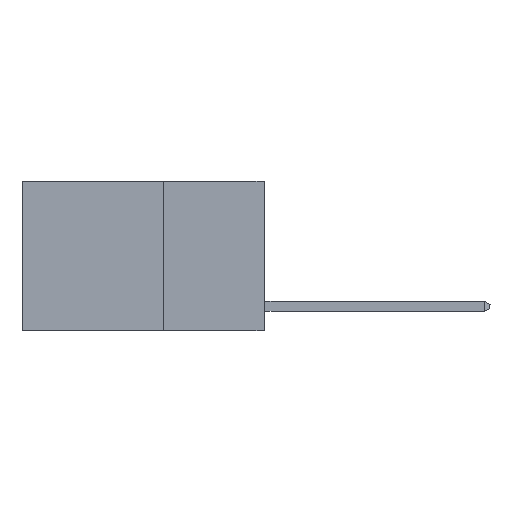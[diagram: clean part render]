
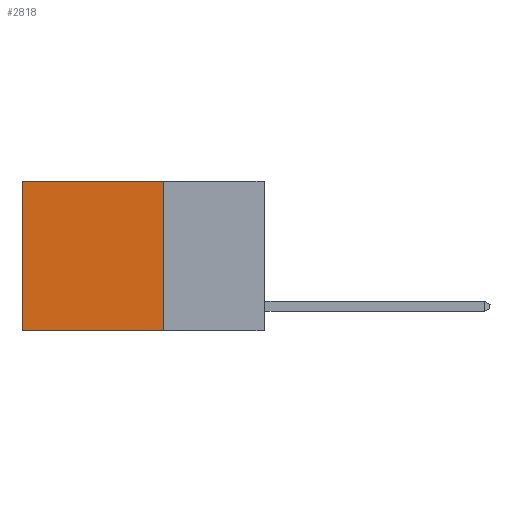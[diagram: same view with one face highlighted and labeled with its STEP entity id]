
A CAD part, left-side view. The second image highlights one B-rep face of the part: STEP entity #2818.
In plain terms, the highlighted planar face has unit normal (-1, 0, 0).
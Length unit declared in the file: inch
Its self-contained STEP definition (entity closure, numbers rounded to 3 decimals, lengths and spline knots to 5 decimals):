
#134 = VECTOR ( 'NONE', #1135, 39.37008 ) ;
#278 = VERTEX_POINT ( 'NONE', #2624 ) ;
#439 = EDGE_CURVE ( 'NONE', #278, #7515, #12090, .T. ) ;
#1135 = DIRECTION ( 'NONE',  ( 0., 1., 0. ) ) ;
#1169 = DIRECTION ( 'NONE',  ( 0., 0., -1. ) ) ;
#2047 = CARTESIAN_POINT ( 'NONE',  ( 0.2625, 0.6, 0. ) ) ;
#2213 = CARTESIAN_POINT ( 'NONE',  ( 0.2625, 0.25, -0.37 ) ) ;
#2285 = ORIENTED_EDGE ( 'NONE', *, *, #439, .F. ) ;
#2624 = CARTESIAN_POINT ( 'NONE',  ( 0.2625, 0.25, -0.37 ) ) ;
#2818 = ADVANCED_FACE ( 'NONE', ( #10756 ), #8108, .F. ) ;
#3013 = VECTOR ( 'NONE', #17238, 39.37008 ) ;
#3111 = VERTEX_POINT ( 'NONE', #2047 ) ;
#3143 = ORIENTED_EDGE ( 'NONE', *, *, #16638, .T. ) ;
#3815 = CARTESIAN_POINT ( 'NONE',  ( 0.2625, 0.25, 0. ) ) ;
#5199 = CARTESIAN_POINT ( 'NONE',  ( 0.2625, 0.25, 0. ) ) ;
#5570 = EDGE_LOOP ( 'NONE', ( #3143, #2285, #6544, #8696 ) ) ;
#6138 = AXIS2_PLACEMENT_3D ( 'NONE', #5199, #16607, #16341 ) ;
#6544 = ORIENTED_EDGE ( 'NONE', *, *, #11732, .F. ) ;
#7515 = VERTEX_POINT ( 'NONE', #16007 ) ;
#8108 = PLANE ( 'NONE',  #6138 ) ;
#8696 = ORIENTED_EDGE ( 'NONE', *, *, #10519, .T. ) ;
#9375 = DIRECTION ( 'NONE',  ( 0., 1., 0. ) ) ;
#10280 = LINE ( 'NONE', #11666, #3013 ) ;
#10519 = EDGE_CURVE ( 'NONE', #14556, #3111, #14672, .T. ) ;
#10756 = FACE_OUTER_BOUND ( 'NONE', #5570, .T. ) ;
#11666 = CARTESIAN_POINT ( 'NONE',  ( 0.2625, 0.6, 0. ) ) ;
#11732 = EDGE_CURVE ( 'NONE', #14556, #278, #17517, .T. ) ;
#12090 = LINE ( 'NONE', #2213, #134 ) ;
#13709 = VECTOR ( 'NONE', #1169, 39.37008 ) ;
#14556 = VERTEX_POINT ( 'NONE', #17639 ) ;
#14672 = LINE ( 'NONE', #3815, #15419 ) ;
#14953 = CARTESIAN_POINT ( 'NONE',  ( 0.2625, 0.25, 0. ) ) ;
#15419 = VECTOR ( 'NONE', #9375, 39.37008 ) ;
#16007 = CARTESIAN_POINT ( 'NONE',  ( 0.2625, 0.6, -0.37 ) ) ;
#16341 = DIRECTION ( 'NONE',  ( 0., 0., -1. ) ) ;
#16607 = DIRECTION ( 'NONE',  ( 1., 0., 0. ) ) ;
#16638 = EDGE_CURVE ( 'NONE', #3111, #7515, #10280, .T. ) ;
#17238 = DIRECTION ( 'NONE',  ( 0., 0., -1. ) ) ;
#17517 = LINE ( 'NONE', #14953, #13709 ) ;
#17639 = CARTESIAN_POINT ( 'NONE',  ( 0.2625, 0.25, 0. ) ) ;
